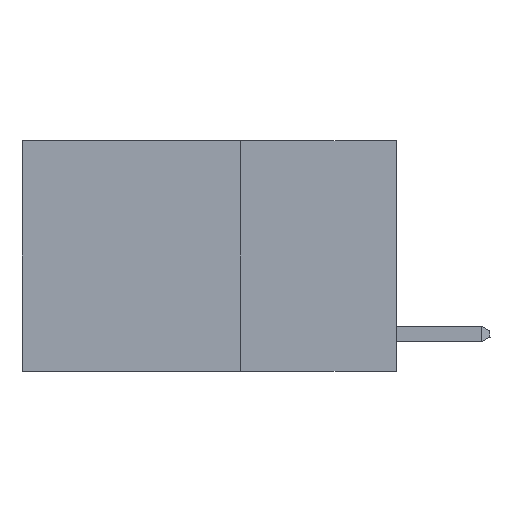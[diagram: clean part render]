
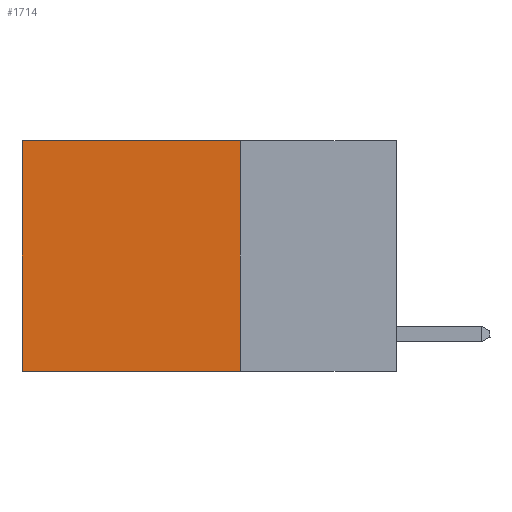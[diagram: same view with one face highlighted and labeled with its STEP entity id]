
A CAD part, left-side view. The second image highlights one B-rep face of the part: STEP entity #1714.
In plain terms, the highlighted planar face has unit normal (-1, 0, 0).
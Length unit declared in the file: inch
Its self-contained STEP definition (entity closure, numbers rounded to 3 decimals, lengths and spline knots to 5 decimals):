
#71 = LINE ( 'NONE', #10323, #23044 ) ;
#1714 = ADVANCED_FACE ( 'NONE', ( #22055 ), #21388, .F. ) ;
#2505 = DIRECTION ( 'NONE',  ( 0., 1., 0. ) ) ;
#4491 = VERTEX_POINT ( 'NONE', #17312 ) ;
#5056 = DIRECTION ( 'NONE',  ( 0., 0., -1. ) ) ;
#5775 = VERTEX_POINT ( 'NONE', #14491 ) ;
#5937 = DIRECTION ( 'NONE',  ( 0., 0., -1. ) ) ;
#5980 = VECTOR ( 'NONE', #12237, 39.37008 ) ;
#7384 = VERTEX_POINT ( 'NONE', #19932 ) ;
#10323 = CARTESIAN_POINT ( 'NONE',  ( 0.2625, 0.25, 0. ) ) ;
#11481 = EDGE_CURVE ( 'NONE', #20164, #7384, #13469, .T. ) ;
#11757 = ORIENTED_EDGE ( 'NONE', *, *, #22355, .F. ) ;
#12237 = DIRECTION ( 'NONE',  ( 0., 1., 0. ) ) ;
#12587 = DIRECTION ( 'NONE',  ( 1., 0., 0. ) ) ;
#12593 = EDGE_LOOP ( 'NONE', ( #27022, #11757, #14375, #18576 ) ) ;
#13469 = LINE ( 'NONE', #13647, #24506 ) ;
#13647 = CARTESIAN_POINT ( 'NONE',  ( 0.2625, 0.25, 0. ) ) ;
#14375 = ORIENTED_EDGE ( 'NONE', *, *, #18624, .F. ) ;
#14491 = CARTESIAN_POINT ( 'NONE',  ( 0.2625, 0.6, -0.37 ) ) ;
#15126 = EDGE_CURVE ( 'NONE', #7384, #5775, #16676, .T. ) ;
#16676 = LINE ( 'NONE', #18330, #28391 ) ;
#17312 = CARTESIAN_POINT ( 'NONE',  ( 0.2625, 0.25, -0.37 ) ) ;
#17682 = CARTESIAN_POINT ( 'NONE',  ( 0.2625, 0.25, 0. ) ) ;
#17761 = LINE ( 'NONE', #27630, #5980 ) ;
#18330 = CARTESIAN_POINT ( 'NONE',  ( 0.2625, 0.6, 0. ) ) ;
#18576 = ORIENTED_EDGE ( 'NONE', *, *, #11481, .T. ) ;
#18624 = EDGE_CURVE ( 'NONE', #20164, #4491, #71, .T. ) ;
#19932 = CARTESIAN_POINT ( 'NONE',  ( 0.2625, 0.6, 0. ) ) ;
#20164 = VERTEX_POINT ( 'NONE', #17682 ) ;
#21388 = PLANE ( 'NONE',  #26949 ) ;
#22055 = FACE_OUTER_BOUND ( 'NONE', #12593, .T. ) ;
#22355 = EDGE_CURVE ( 'NONE', #4491, #5775, #17761, .T. ) ;
#23044 = VECTOR ( 'NONE', #5937, 39.37008 ) ;
#24506 = VECTOR ( 'NONE', #2505, 39.37008 ) ;
#25799 = CARTESIAN_POINT ( 'NONE',  ( 0.2625, 0.25, 0. ) ) ;
#26949 = AXIS2_PLACEMENT_3D ( 'NONE', #25799, #12587, #27984 ) ;
#27022 = ORIENTED_EDGE ( 'NONE', *, *, #15126, .T. ) ;
#27630 = CARTESIAN_POINT ( 'NONE',  ( 0.2625, 0.25, -0.37 ) ) ;
#27984 = DIRECTION ( 'NONE',  ( 0., 0., -1. ) ) ;
#28391 = VECTOR ( 'NONE', #5056, 39.37008 ) ;
